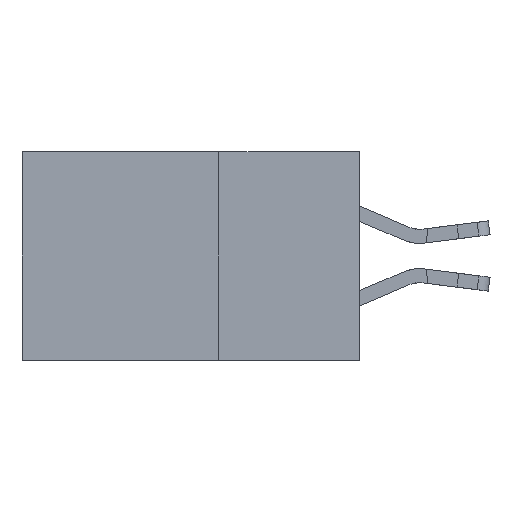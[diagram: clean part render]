
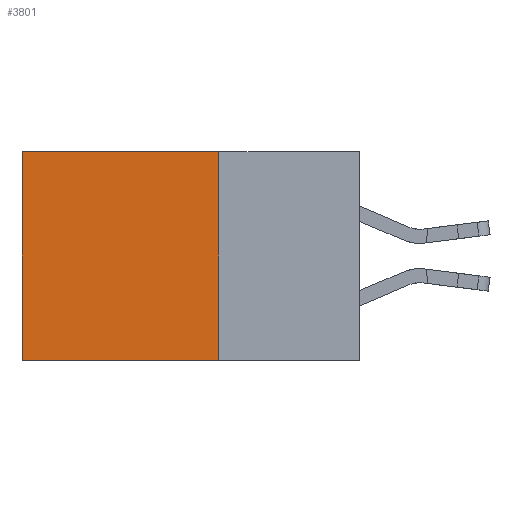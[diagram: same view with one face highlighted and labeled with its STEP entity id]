
A CAD part, left-side view. The second image highlights one B-rep face of the part: STEP entity #3801.
In plain terms, the highlighted planar face has unit normal (-1, 0, 0).
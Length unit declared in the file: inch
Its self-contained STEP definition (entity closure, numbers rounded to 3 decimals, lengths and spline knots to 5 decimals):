
#102 = EDGE_CURVE ( 'NONE', #14469, #7006, #9626, .T. ) ;
#463 = CARTESIAN_POINT ( 'NONE',  ( 0.2875, 0.25, -0.37 ) ) ;
#528 = ORIENTED_EDGE ( 'NONE', *, *, #102, .T. ) ;
#1608 = EDGE_CURVE ( 'NONE', #10784, #10034, #16044, .T. ) ;
#2242 = DIRECTION ( 'NONE',  ( 0., 1., 0. ) ) ;
#2391 = CARTESIAN_POINT ( 'NONE',  ( 0.2875, 0.25, 0. ) ) ;
#2793 = VECTOR ( 'NONE', #2242, 39.37008 ) ;
#3527 = DIRECTION ( 'NONE',  ( 0., 0., -1. ) ) ;
#3801 = ADVANCED_FACE ( 'NONE', ( #10502 ), #8408, .F. ) ;
#4450 = EDGE_LOOP ( 'NONE', ( #4741, #13898, #9095, #528 ) ) ;
#4727 = DIRECTION ( 'NONE',  ( 0., 0., -1. ) ) ;
#4741 = ORIENTED_EDGE ( 'NONE', *, *, #12714, .T. ) ;
#4908 = DIRECTION ( 'NONE',  ( 0., 0., -1. ) ) ;
#5197 = AXIS2_PLACEMENT_3D ( 'NONE', #8425, #8298, #4727 ) ;
#6164 = VECTOR ( 'NONE', #11674, 39.37008 ) ;
#7006 = VERTEX_POINT ( 'NONE', #15413 ) ;
#7396 = CARTESIAN_POINT ( 'NONE',  ( 0.2875, 0.6, 0. ) ) ;
#8094 = CARTESIAN_POINT ( 'NONE',  ( 0.2875, 0.25, -0.37 ) ) ;
#8249 = VECTOR ( 'NONE', #3527, 39.37008 ) ;
#8298 = DIRECTION ( 'NONE',  ( 1., 0., 0. ) ) ;
#8408 = PLANE ( 'NONE',  #5197 ) ;
#8425 = CARTESIAN_POINT ( 'NONE',  ( 0.2875, 0.25, 0. ) ) ;
#8440 = VECTOR ( 'NONE', #4908, 39.37008 ) ;
#9095 = ORIENTED_EDGE ( 'NONE', *, *, #10005, .F. ) ;
#9626 = LINE ( 'NONE', #2391, #2793 ) ;
#10005 = EDGE_CURVE ( 'NONE', #14469, #10784, #11748, .T. ) ;
#10029 = CARTESIAN_POINT ( 'NONE',  ( 0.2875, 0.6, -0.37 ) ) ;
#10034 = VERTEX_POINT ( 'NONE', #10029 ) ;
#10502 = FACE_OUTER_BOUND ( 'NONE', #4450, .T. ) ;
#10718 = CARTESIAN_POINT ( 'NONE',  ( 0.2875, 0.25, 0. ) ) ;
#10784 = VERTEX_POINT ( 'NONE', #463 ) ;
#11590 = LINE ( 'NONE', #7396, #8249 ) ;
#11674 = DIRECTION ( 'NONE',  ( 0., 1., 0. ) ) ;
#11748 = LINE ( 'NONE', #13668, #8440 ) ;
#12714 = EDGE_CURVE ( 'NONE', #7006, #10034, #11590, .T. ) ;
#13668 = CARTESIAN_POINT ( 'NONE',  ( 0.2875, 0.25, 0. ) ) ;
#13898 = ORIENTED_EDGE ( 'NONE', *, *, #1608, .F. ) ;
#14469 = VERTEX_POINT ( 'NONE', #10718 ) ;
#15413 = CARTESIAN_POINT ( 'NONE',  ( 0.2875, 0.6, 0. ) ) ;
#16044 = LINE ( 'NONE', #8094, #6164 ) ;
